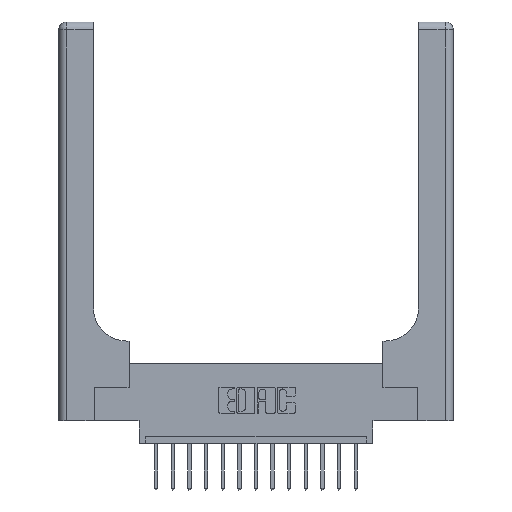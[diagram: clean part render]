
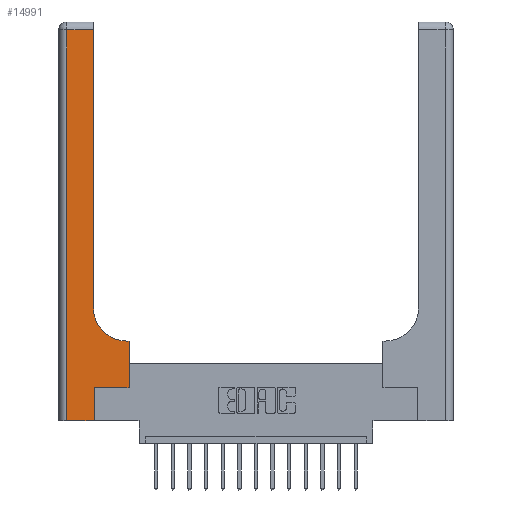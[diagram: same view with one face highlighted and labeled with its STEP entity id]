
A CAD part, top view. The second image highlights one B-rep face of the part: STEP entity #14991.
In plain terms, the highlighted planar face has unit normal (0, 0, 1).
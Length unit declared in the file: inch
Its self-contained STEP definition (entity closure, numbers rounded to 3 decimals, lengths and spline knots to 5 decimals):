
#207 = VERTEX_POINT ( 'NONE', #3595 ) ;
#424 = PLANE ( 'NONE',  #13008 ) ;
#556 = CARTESIAN_POINT ( 'NONE',  ( 0.26, 2.94, 0.37 ) ) ;
#569 = ORIENTED_EDGE ( 'NONE', *, *, #13482, .T. ) ;
#1204 = CARTESIAN_POINT ( 'NONE',  ( 0.265, 0., 0.37 ) ) ;
#1441 = LINE ( 'NONE', #6907, #2988 ) ;
#1513 = VECTOR ( 'NONE', #2635, 39.37008 ) ;
#1724 = CARTESIAN_POINT ( 'NONE',  ( 0.06, 2.94, 0.37 ) ) ;
#2050 = VECTOR ( 'NONE', #5045, 39.37008 ) ;
#2229 = EDGE_CURVE ( 'NONE', #7415, #17445, #3806, .T. ) ;
#2390 = ORIENTED_EDGE ( 'NONE', *, *, #12020, .T. ) ;
#2536 = EDGE_CURVE ( 'NONE', #17445, #16483, #1441, .T. ) ;
#2635 = DIRECTION ( 'NONE',  ( 0., 1., 0. ) ) ;
#2829 = ORIENTED_EDGE ( 'NONE', *, *, #12764, .T. ) ;
#2988 = VECTOR ( 'NONE', #7175, 39.37008 ) ;
#3017 = VERTEX_POINT ( 'NONE', #556 ) ;
#3147 = ORIENTED_EDGE ( 'NONE', *, *, #8616, .T. ) ;
#3202 = DIRECTION ( 'NONE',  ( 0., 0., -1. ) ) ;
#3488 = ORIENTED_EDGE ( 'NONE', *, *, #2229, .T. ) ;
#3546 = EDGE_CURVE ( 'NONE', #5314, #207, #17527, .T. ) ;
#3595 = CARTESIAN_POINT ( 'NONE',  ( 0.06, 0., 0.37 ) ) ;
#3615 = ORIENTED_EDGE ( 'NONE', *, *, #15946, .T. ) ;
#3672 = LINE ( 'NONE', #5265, #14649 ) ;
#3758 = ORIENTED_EDGE ( 'NONE', *, *, #3546, .T. ) ;
#3806 = LINE ( 'NONE', #1204, #6236 ) ;
#4104 = DIRECTION ( 'NONE',  ( 0., 1., 0. ) ) ;
#4851 = AXIS2_PLACEMENT_3D ( 'NONE', #12551, #3202, #14160 ) ;
#5045 = DIRECTION ( 'NONE',  ( -1., 0., 0. ) ) ;
#5265 = CARTESIAN_POINT ( 'NONE',  ( 0.528, 0.25, 0.37 ) ) ;
#5314 = VERTEX_POINT ( 'NONE', #1724 ) ;
#5389 = DIRECTION ( 'NONE',  ( 1., 0., 0. ) ) ;
#5664 = LINE ( 'NONE', #17697, #13883 ) ;
#5900 = CARTESIAN_POINT ( 'NONE',  ( 0., 3., 0.37 ) ) ;
#6236 = VECTOR ( 'NONE', #14667, 39.37008 ) ;
#6581 = CARTESIAN_POINT ( 'NONE',  ( 0.06, 3., 0.37 ) ) ;
#6875 = DIRECTION ( 'NONE',  ( -1., 0., 0. ) ) ;
#6907 = CARTESIAN_POINT ( 'NONE',  ( 0.265, 0.25, 0.37 ) ) ;
#6947 = ORIENTED_EDGE ( 'NONE', *, *, #10969, .T. ) ;
#7175 = DIRECTION ( 'NONE',  ( 1., 0., 0. ) ) ;
#7415 = VERTEX_POINT ( 'NONE', #9665 ) ;
#7773 = CARTESIAN_POINT ( 'NONE',  ( 0.528, 0.25, 0.37 ) ) ;
#7959 = VECTOR ( 'NONE', #10639, 39.37008 ) ;
#8517 = LINE ( 'NONE', #11305, #10948 ) ;
#8616 = EDGE_CURVE ( 'NONE', #17701, #8762, #9434, .T. ) ;
#8762 = VERTEX_POINT ( 'NONE', #10553 ) ;
#8810 = CARTESIAN_POINT ( 'NONE',  ( 0.51, 0.6, 0.37 ) ) ;
#9388 = LINE ( 'NONE', #14857, #1513 ) ;
#9434 = CIRCLE ( 'NONE', #4851, 0.25 ) ;
#9665 = CARTESIAN_POINT ( 'NONE',  ( 0.265, 0., 0.37 ) ) ;
#10434 = CARTESIAN_POINT ( 'NONE',  ( 0.265, 0.25, 0.37 ) ) ;
#10437 = VERTEX_POINT ( 'NONE', #10802 ) ;
#10553 = CARTESIAN_POINT ( 'NONE',  ( 0.26, 0.85, 0.37 ) ) ;
#10639 = DIRECTION ( 'NONE',  ( 0., -1., 0. ) ) ;
#10802 = CARTESIAN_POINT ( 'NONE',  ( 0.528, 0.6, 0.37 ) ) ;
#10806 = LINE ( 'NONE', #14660, #2050 ) ;
#10948 = VECTOR ( 'NONE', #13796, 39.37008 ) ;
#10969 = EDGE_CURVE ( 'NONE', #3017, #5314, #8517, .T. ) ;
#11305 = CARTESIAN_POINT ( 'NONE',  ( 0., 2.94, 0.37 ) ) ;
#12020 = EDGE_CURVE ( 'NONE', #16483, #10437, #3672, .T. ) ;
#12551 = CARTESIAN_POINT ( 'NONE',  ( 0.51, 0.85, 0.37 ) ) ;
#12730 = DIRECTION ( 'NONE',  ( 0., 0., -1. ) ) ;
#12764 = EDGE_CURVE ( 'NONE', #10437, #17701, #10806, .T. ) ;
#13008 = AXIS2_PLACEMENT_3D ( 'NONE', #5900, #12730, #6875 ) ;
#13482 = EDGE_CURVE ( 'NONE', #8762, #3017, #9388, .T. ) ;
#13796 = DIRECTION ( 'NONE',  ( -1., 0., 0. ) ) ;
#13883 = VECTOR ( 'NONE', #5389, 39.37008 ) ;
#14160 = DIRECTION ( 'NONE',  ( 1., 0., 0. ) ) ;
#14649 = VECTOR ( 'NONE', #4104, 39.37008 ) ;
#14660 = CARTESIAN_POINT ( 'NONE',  ( 0.26, 0.6, 0.37 ) ) ;
#14667 = DIRECTION ( 'NONE',  ( 0., 1., 0. ) ) ;
#14857 = CARTESIAN_POINT ( 'NONE',  ( 0.26, 3., 0.37 ) ) ;
#14991 = ADVANCED_FACE ( 'NONE', ( #15134 ), #424, .F. ) ;
#15134 = FACE_OUTER_BOUND ( 'NONE', #15886, .T. ) ;
#15886 = EDGE_LOOP ( 'NONE', ( #569, #6947, #3758, #3615, #3488, #16736, #2390, #2829, #3147 ) ) ;
#15946 = EDGE_CURVE ( 'NONE', #207, #7415, #5664, .T. ) ;
#16483 = VERTEX_POINT ( 'NONE', #7773 ) ;
#16736 = ORIENTED_EDGE ( 'NONE', *, *, #2536, .T. ) ;
#17445 = VERTEX_POINT ( 'NONE', #10434 ) ;
#17527 = LINE ( 'NONE', #6581, #7959 ) ;
#17697 = CARTESIAN_POINT ( 'NONE',  ( 0., 0., 0.37 ) ) ;
#17701 = VERTEX_POINT ( 'NONE', #8810 ) ;
